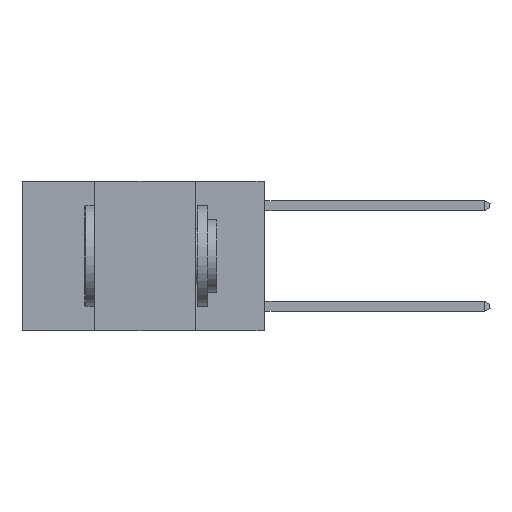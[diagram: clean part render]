
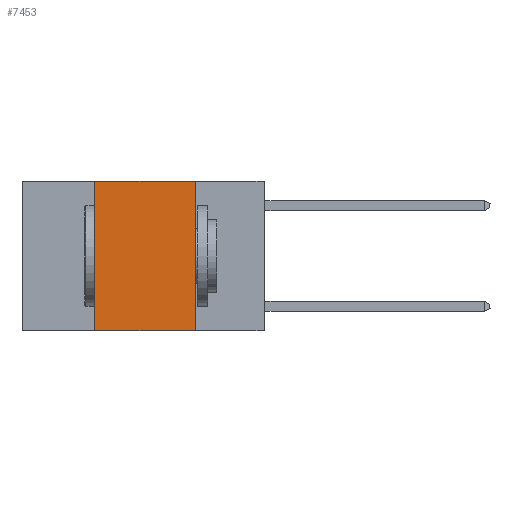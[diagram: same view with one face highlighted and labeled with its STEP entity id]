
A CAD part, left-side view. The second image highlights one B-rep face of the part: STEP entity #7453.
In plain terms, the highlighted planar face has unit normal (-1, 0, 0).
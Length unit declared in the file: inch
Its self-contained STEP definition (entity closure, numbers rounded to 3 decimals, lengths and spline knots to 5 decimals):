
#339 = VECTOR ( 'NONE', #13474, 39.37008 ) ;
#516 = CARTESIAN_POINT ( 'NONE',  ( 0., 0.17, -0.37 ) ) ;
#559 = CARTESIAN_POINT ( 'NONE',  ( 0., 0.42, 0. ) ) ;
#689 = VERTEX_POINT ( 'NONE', #9158 ) ;
#848 = LINE ( 'NONE', #3017, #11084 ) ;
#1268 = VERTEX_POINT ( 'NONE', #559 ) ;
#1374 = DIRECTION ( 'NONE',  ( 0., 0., -1. ) ) ;
#1635 = DIRECTION ( 'NONE',  ( 0., -1., 0. ) ) ;
#2154 = EDGE_LOOP ( 'NONE', ( #12226, #8041, #4631, #2240 ) ) ;
#2169 = VECTOR ( 'NONE', #8607, 39.37008 ) ;
#2240 = ORIENTED_EDGE ( 'NONE', *, *, #5900, .T. ) ;
#2502 = DIRECTION ( 'NONE',  ( 1., 0., 0. ) ) ;
#2972 = EDGE_CURVE ( 'NONE', #689, #9624, #5488, .T. ) ;
#3017 = CARTESIAN_POINT ( 'NONE',  ( 0., 0.6, -0.37 ) ) ;
#3599 = FACE_OUTER_BOUND ( 'NONE', #2154, .T. ) ;
#3988 = CARTESIAN_POINT ( 'NONE',  ( 0., 0.42, 0. ) ) ;
#4135 = EDGE_CURVE ( 'NONE', #1268, #689, #8393, .T. ) ;
#4352 = DIRECTION ( 'NONE',  ( 0., -1., 0. ) ) ;
#4631 = ORIENTED_EDGE ( 'NONE', *, *, #14104, .F. ) ;
#5488 = LINE ( 'NONE', #9926, #339 ) ;
#5900 = EDGE_CURVE ( 'NONE', #13602, #9624, #848, .T. ) ;
#6317 = VECTOR ( 'NONE', #1635, 39.37008 ) ;
#7267 = CARTESIAN_POINT ( 'NONE',  ( 0., 0.6, 0. ) ) ;
#7453 = ADVANCED_FACE ( 'NONE', ( #3599 ), #8142, .F. ) ;
#8041 = ORIENTED_EDGE ( 'NONE', *, *, #4135, .F. ) ;
#8142 = PLANE ( 'NONE',  #9889 ) ;
#8393 = LINE ( 'NONE', #7267, #6317 ) ;
#8607 = DIRECTION ( 'NONE',  ( 0., 0., 1. ) ) ;
#9158 = CARTESIAN_POINT ( 'NONE',  ( 0., 0.17, 0. ) ) ;
#9624 = VERTEX_POINT ( 'NONE', #516 ) ;
#9646 = LINE ( 'NONE', #3988, #2169 ) ;
#9889 = AXIS2_PLACEMENT_3D ( 'NONE', #12644, #2502, #1374 ) ;
#9926 = CARTESIAN_POINT ( 'NONE',  ( 0., 0.17, 0. ) ) ;
#11084 = VECTOR ( 'NONE', #4352, 39.37008 ) ;
#12082 = CARTESIAN_POINT ( 'NONE',  ( 0., 0.42, -0.37 ) ) ;
#12226 = ORIENTED_EDGE ( 'NONE', *, *, #2972, .F. ) ;
#12644 = CARTESIAN_POINT ( 'NONE',  ( 0., 0.6, 0. ) ) ;
#13474 = DIRECTION ( 'NONE',  ( 0., 0., -1. ) ) ;
#13602 = VERTEX_POINT ( 'NONE', #12082 ) ;
#14104 = EDGE_CURVE ( 'NONE', #13602, #1268, #9646, .T. ) ;
